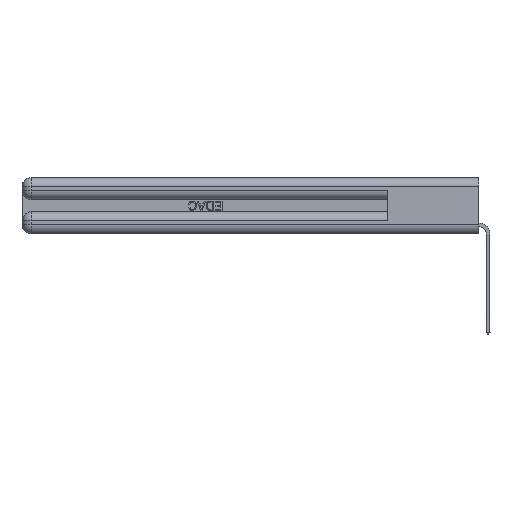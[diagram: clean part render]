
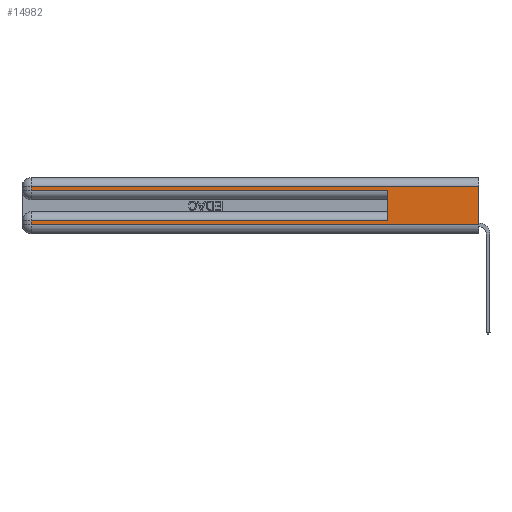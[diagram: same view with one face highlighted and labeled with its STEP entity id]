
A CAD part, left-side view. The second image highlights one B-rep face of the part: STEP entity #14982.
In plain terms, the highlighted planar face has unit normal (-1, 0, 0).
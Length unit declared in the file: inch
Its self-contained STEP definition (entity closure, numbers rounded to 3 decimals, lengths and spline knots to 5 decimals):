
#188 = ORIENTED_EDGE ( 'NONE', *, *, #25834, .F. ) ;
#700 = EDGE_LOOP ( 'NONE', ( #23950, #31696, #23455, #1470, #188, #3776, #3096, #8094 ) ) ;
#734 = VECTOR ( 'NONE', #30468, 39.37008 ) ;
#1470 = ORIENTED_EDGE ( 'NONE', *, *, #20871, .T. ) ;
#1630 = VERTEX_POINT ( 'NONE', #30393 ) ;
#1932 = VECTOR ( 'NONE', #24755, 39.37008 ) ;
#2153 = CARTESIAN_POINT ( 'NONE',  ( 0., 0., 0.31 ) ) ;
#2385 = CARTESIAN_POINT ( 'NONE',  ( 0., 0., 0.06 ) ) ;
#3096 = ORIENTED_EDGE ( 'NONE', *, *, #8944, .T. ) ;
#3594 = CARTESIAN_POINT ( 'NONE',  ( 0., 2.94, 0.285 ) ) ;
#3719 = EDGE_CURVE ( 'NONE', #7942, #14133, #7537, .T. ) ;
#3776 = ORIENTED_EDGE ( 'NONE', *, *, #3719, .T. ) ;
#6086 = AXIS2_PLACEMENT_3D ( 'NONE', #16861, #26683, #12072 ) ;
#6590 = CARTESIAN_POINT ( 'NONE',  ( 0., 0.6, 0.085 ) ) ;
#6887 = LINE ( 'NONE', #21071, #19144 ) ;
#7123 = LINE ( 'NONE', #28894, #12107 ) ;
#7537 = LINE ( 'NONE', #17522, #19779 ) ;
#7942 = VERTEX_POINT ( 'NONE', #6590 ) ;
#8094 = ORIENTED_EDGE ( 'NONE', *, *, #19473, .T. ) ;
#8602 = LINE ( 'NONE', #15006, #1932 ) ;
#8944 = EDGE_CURVE ( 'NONE', #14133, #27665, #15925, .T. ) ;
#12072 = DIRECTION ( 'NONE',  ( 0., 0., -1. ) ) ;
#12107 = VECTOR ( 'NONE', #21624, 39.37008 ) ;
#13386 = CARTESIAN_POINT ( 'NONE',  ( 0., 2.94, 0.37 ) ) ;
#13477 = LINE ( 'NONE', #27526, #25696 ) ;
#13765 = EDGE_CURVE ( 'NONE', #25447, #1630, #7123, .T. ) ;
#14133 = VERTEX_POINT ( 'NONE', #30872 ) ;
#14982 = ADVANCED_FACE ( 'NONE', ( #16595 ), #24242, .F. ) ;
#14997 = VERTEX_POINT ( 'NONE', #31567 ) ;
#15006 = CARTESIAN_POINT ( 'NONE',  ( 0., 2.94, 0.37 ) ) ;
#15807 = DIRECTION ( 'NONE',  ( 0., 0., -1. ) ) ;
#15827 = CARTESIAN_POINT ( 'NONE',  ( 0., 0.6, 0.145 ) ) ;
#15925 = LINE ( 'NONE', #13386, #28167 ) ;
#16595 = FACE_OUTER_BOUND ( 'NONE', #700, .T. ) ;
#16861 = CARTESIAN_POINT ( 'NONE',  ( 0., 0., 0.37 ) ) ;
#16942 = EDGE_CURVE ( 'NONE', #25447, #14997, #6887, .T. ) ;
#17522 = CARTESIAN_POINT ( 'NONE',  ( 0., 0., 0.085 ) ) ;
#19144 = VECTOR ( 'NONE', #23533, 39.37008 ) ;
#19473 = EDGE_CURVE ( 'NONE', #27665, #1630, #27801, .T. ) ;
#19779 = VECTOR ( 'NONE', #22426, 39.37008 ) ;
#20400 = CARTESIAN_POINT ( 'NONE',  ( 0., 0.6, 0.285 ) ) ;
#20427 = LINE ( 'NONE', #15827, #734 ) ;
#20871 = EDGE_CURVE ( 'NONE', #26988, #22330, #13477, .T. ) ;
#21071 = CARTESIAN_POINT ( 'NONE',  ( 0., 0., 0.31 ) ) ;
#21319 = VECTOR ( 'NONE', #22063, 39.37008 ) ;
#21624 = DIRECTION ( 'NONE',  ( 0., 0., -1. ) ) ;
#22063 = DIRECTION ( 'NONE',  ( 0., -1., 0. ) ) ;
#22330 = VERTEX_POINT ( 'NONE', #20400 ) ;
#22426 = DIRECTION ( 'NONE',  ( 0., 1., 0. ) ) ;
#23455 = ORIENTED_EDGE ( 'NONE', *, *, #25595, .T. ) ;
#23533 = DIRECTION ( 'NONE',  ( 0., 1., 0. ) ) ;
#23950 = ORIENTED_EDGE ( 'NONE', *, *, #13765, .F. ) ;
#24242 = PLANE ( 'NONE',  #6086 ) ;
#24755 = DIRECTION ( 'NONE',  ( 0., 0., -1. ) ) ;
#25447 = VERTEX_POINT ( 'NONE', #2153 ) ;
#25595 = EDGE_CURVE ( 'NONE', #14997, #26988, #8602, .T. ) ;
#25696 = VECTOR ( 'NONE', #29993, 39.37008 ) ;
#25834 = EDGE_CURVE ( 'NONE', #7942, #22330, #20427, .T. ) ;
#26683 = DIRECTION ( 'NONE',  ( 1., 0., 0. ) ) ;
#26988 = VERTEX_POINT ( 'NONE', #3594 ) ;
#27526 = CARTESIAN_POINT ( 'NONE',  ( 0., 0., 0.285 ) ) ;
#27665 = VERTEX_POINT ( 'NONE', #27979 ) ;
#27801 = LINE ( 'NONE', #2385, #21319 ) ;
#27979 = CARTESIAN_POINT ( 'NONE',  ( 0., 2.94, 0.06 ) ) ;
#28167 = VECTOR ( 'NONE', #15807, 39.37008 ) ;
#28894 = CARTESIAN_POINT ( 'NONE',  ( 0., 0., 0.37 ) ) ;
#29993 = DIRECTION ( 'NONE',  ( 0., -1., 0. ) ) ;
#30393 = CARTESIAN_POINT ( 'NONE',  ( 0., 0., 0.06 ) ) ;
#30468 = DIRECTION ( 'NONE',  ( 0., 0., 1. ) ) ;
#30872 = CARTESIAN_POINT ( 'NONE',  ( 0., 2.94, 0.085 ) ) ;
#31567 = CARTESIAN_POINT ( 'NONE',  ( 0., 2.94, 0.31 ) ) ;
#31696 = ORIENTED_EDGE ( 'NONE', *, *, #16942, .T. ) ;
